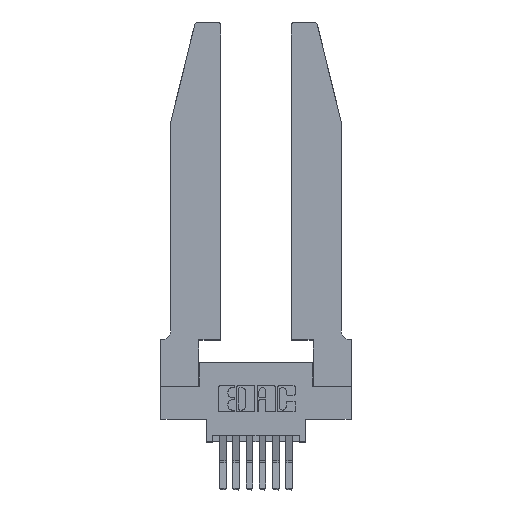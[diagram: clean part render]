
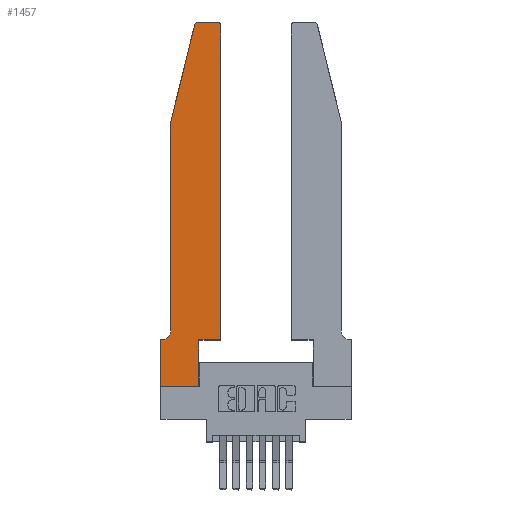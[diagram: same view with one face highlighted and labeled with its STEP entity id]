
A CAD part, top view. The second image highlights one B-rep face of the part: STEP entity #1457.
In plain terms, the highlighted planar face has unit normal (0, 0, 1).
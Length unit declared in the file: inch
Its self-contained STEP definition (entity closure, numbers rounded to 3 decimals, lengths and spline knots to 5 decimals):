
#40 = CARTESIAN_POINT ( 'NONE',  ( 0.2865, 0.35, 0.37 ) ) ;
#270 = VECTOR ( 'NONE', #13440, 39.37008 ) ;
#539 = EDGE_CURVE ( 'NONE', #5631, #12162, #7547, .T. ) ;
#817 = EDGE_CURVE ( 'NONE', #2137, #12603, #7372, .T. ) ;
#1002 = EDGE_CURVE ( 'NONE', #5883, #2137, #11207, .T. ) ;
#1016 = FACE_OUTER_BOUND ( 'NONE', #14484, .T. ) ;
#1052 = AXIS2_PLACEMENT_3D ( 'NONE', #11896, #5185, #13022 ) ;
#1059 = ORIENTED_EDGE ( 'NONE', *, *, #13550, .T. ) ;
#1457 = ADVANCED_FACE ( 'NONE', ( #1016 ), #13391, .T. ) ;
#1832 = CARTESIAN_POINT ( 'NONE',  ( 0., 0., 0.37 ) ) ;
#2078 = CIRCLE ( 'NONE', #1052, 0.03 ) ;
#2098 = DIRECTION ( 'NONE',  ( 0., 0., 1. ) ) ;
#2137 = VERTEX_POINT ( 'NONE', #9943 ) ;
#2771 = EDGE_CURVE ( 'NONE', #5979, #12823, #2805, .T. ) ;
#2805 = LINE ( 'NONE', #4105, #14296 ) ;
#3037 = VECTOR ( 'NONE', #4984, 39.37008 ) ;
#3042 = ORIENTED_EDGE ( 'NONE', *, *, #12965, .T. ) ;
#3043 = LINE ( 'NONE', #6247, #8605 ) ;
#3087 = ORIENTED_EDGE ( 'NONE', *, *, #8734, .T. ) ;
#3694 = CARTESIAN_POINT ( 'NONE',  ( 0.0755, 2., 0.37 ) ) ;
#3719 = DIRECTION ( 'NONE',  ( 0., 0., -1. ) ) ;
#3932 = VERTEX_POINT ( 'NONE', #12540 ) ;
#4089 = ORIENTED_EDGE ( 'NONE', *, *, #817, .T. ) ;
#4105 = CARTESIAN_POINT ( 'NONE',  ( 0.2605, 2.75, 0.37 ) ) ;
#4128 = ORIENTED_EDGE ( 'NONE', *, *, #5196, .T. ) ;
#4588 = DIRECTION ( 'NONE',  ( 0., 1., 0. ) ) ;
#4806 = VECTOR ( 'NONE', #6702, 39.37008 ) ;
#4925 = VECTOR ( 'NONE', #13739, 39.37008 ) ;
#4984 = DIRECTION ( 'NONE',  ( 1., 0., 0. ) ) ;
#5185 = DIRECTION ( 'NONE',  ( 0., 0., 1. ) ) ;
#5196 = EDGE_CURVE ( 'NONE', #12603, #14358, #13376, .T. ) ;
#5397 = LINE ( 'NONE', #13038, #11345 ) ;
#5611 = CARTESIAN_POINT ( 'NONE',  ( 0.0755, 0.35, 0.37 ) ) ;
#5631 = VERTEX_POINT ( 'NONE', #12059 ) ;
#5692 = CARTESIAN_POINT ( 'NONE',  ( 0.4505, 0.35, 0.37 ) ) ;
#5760 = ORIENTED_EDGE ( 'NONE', *, *, #7942, .T. ) ;
#5883 = VERTEX_POINT ( 'NONE', #6882 ) ;
#5979 = VERTEX_POINT ( 'NONE', #12626 ) ;
#6247 = CARTESIAN_POINT ( 'NONE',  ( 0.0755, 2., 0.37 ) ) ;
#6317 = DIRECTION ( 'NONE',  ( 0., -1., 0. ) ) ;
#6677 = VECTOR ( 'NONE', #7545, 39.37008 ) ;
#6678 = ORIENTED_EDGE ( 'NONE', *, *, #11827, .T. ) ;
#6702 = DIRECTION ( 'NONE',  ( 1., 0., 0. ) ) ;
#6876 = DIRECTION ( 'NONE',  ( -1., 0., 0. ) ) ;
#6882 = CARTESIAN_POINT ( 'NONE',  ( 0., 0., 0.37 ) ) ;
#6892 = EDGE_CURVE ( 'NONE', #14358, #3932, #7042, .T. ) ;
#7042 = LINE ( 'NONE', #9741, #6677 ) ;
#7162 = CIRCLE ( 'NONE', #13261, 0.07 ) ;
#7372 = LINE ( 'NONE', #9482, #13647 ) ;
#7545 = DIRECTION ( 'NONE',  ( 0., 1., 0. ) ) ;
#7547 = LINE ( 'NONE', #14328, #4925 ) ;
#7942 = EDGE_CURVE ( 'NONE', #12162, #8428, #3043, .T. ) ;
#8428 = VERTEX_POINT ( 'NONE', #12704 ) ;
#8605 = VECTOR ( 'NONE', #11840, 39.37008 ) ;
#8734 = EDGE_CURVE ( 'NONE', #3932, #5979, #13299, .T. ) ;
#8772 = CARTESIAN_POINT ( 'NONE',  ( 0.4205, 2.72, 0.37 ) ) ;
#8900 = LINE ( 'NONE', #5611, #270 ) ;
#9217 = VERTEX_POINT ( 'NONE', #13025 ) ;
#9385 = EDGE_CURVE ( 'NONE', #14176, #9217, #8900, .T. ) ;
#9410 = ORIENTED_EDGE ( 'NONE', *, *, #539, .T. ) ;
#9482 = CARTESIAN_POINT ( 'NONE',  ( 0.2865, 0.35, 0.37 ) ) ;
#9741 = CARTESIAN_POINT ( 'NONE',  ( 0.4505, 0.35, 0.37 ) ) ;
#9898 = DIRECTION ( 'NONE',  ( 1., 0., 0. ) ) ;
#9943 = CARTESIAN_POINT ( 'NONE',  ( 0.2865, 0., 0.37 ) ) ;
#10378 = CARTESIAN_POINT ( 'NONE',  ( 0.0055, 0.42, 0.37 ) ) ;
#11017 = ORIENTED_EDGE ( 'NONE', *, *, #9385, .T. ) ;
#11207 = LINE ( 'NONE', #1832, #3037 ) ;
#11345 = VECTOR ( 'NONE', #6317, 39.37008 ) ;
#11359 = DIRECTION ( 'NONE',  ( 0., 0., 1. ) ) ;
#11527 = DIRECTION ( 'NONE',  ( -1., 0., 0. ) ) ;
#11554 = AXIS2_PLACEMENT_3D ( 'NONE', #8772, #2098, #9898 ) ;
#11657 = DIRECTION ( 'NONE',  ( 1., 0., 0. ) ) ;
#11827 = EDGE_CURVE ( 'NONE', #8428, #14176, #7162, .T. ) ;
#11840 = DIRECTION ( 'NONE',  ( 0., -1., 0. ) ) ;
#11896 = CARTESIAN_POINT ( 'NONE',  ( 0.284, 2.72, 0.37 ) ) ;
#12059 = CARTESIAN_POINT ( 'NONE',  ( 0.25487, 2.72718, 0.37 ) ) ;
#12162 = VERTEX_POINT ( 'NONE', #3694 ) ;
#12503 = CARTESIAN_POINT ( 'NONE',  ( 0.4505, 0.35, 0.37 ) ) ;
#12540 = CARTESIAN_POINT ( 'NONE',  ( 0.4505, 2.72, 0.37 ) ) ;
#12562 = ORIENTED_EDGE ( 'NONE', *, *, #2771, .T. ) ;
#12603 = VERTEX_POINT ( 'NONE', #40 ) ;
#12626 = CARTESIAN_POINT ( 'NONE',  ( 0.4205, 2.75, 0.37 ) ) ;
#12663 = ORIENTED_EDGE ( 'NONE', *, *, #1002, .T. ) ;
#12704 = CARTESIAN_POINT ( 'NONE',  ( 0.0755, 0.42, 0.37 ) ) ;
#12800 = CARTESIAN_POINT ( 'NONE',  ( 0.284, 2.75, 0.37 ) ) ;
#12823 = VERTEX_POINT ( 'NONE', #12800 ) ;
#12965 = EDGE_CURVE ( 'NONE', #9217, #5883, #5397, .T. ) ;
#13022 = DIRECTION ( 'NONE',  ( 1., 0., 0. ) ) ;
#13025 = CARTESIAN_POINT ( 'NONE',  ( 0., 0.35, 0.37 ) ) ;
#13038 = CARTESIAN_POINT ( 'NONE',  ( 0., 0., 0.37 ) ) ;
#13241 = ORIENTED_EDGE ( 'NONE', *, *, #6892, .T. ) ;
#13261 = AXIS2_PLACEMENT_3D ( 'NONE', #10378, #3719, #11527 ) ;
#13299 = CIRCLE ( 'NONE', #11554, 0.03 ) ;
#13376 = LINE ( 'NONE', #12503, #4806 ) ;
#13391 = PLANE ( 'NONE',  #13435 ) ;
#13435 = AXIS2_PLACEMENT_3D ( 'NONE', #13439, #11359, #11657 ) ;
#13439 = CARTESIAN_POINT ( 'NONE',  ( 0., 0.35, 0.37 ) ) ;
#13440 = DIRECTION ( 'NONE',  ( -1., 0., 0. ) ) ;
#13550 = EDGE_CURVE ( 'NONE', #12823, #5631, #2078, .T. ) ;
#13647 = VECTOR ( 'NONE', #4588, 39.37008 ) ;
#13739 = DIRECTION ( 'NONE',  ( -0.239, -0.971, 0. ) ) ;
#14107 = CARTESIAN_POINT ( 'NONE',  ( 0.0055, 0.35, 0.37 ) ) ;
#14176 = VERTEX_POINT ( 'NONE', #14107 ) ;
#14296 = VECTOR ( 'NONE', #6876, 39.37008 ) ;
#14328 = CARTESIAN_POINT ( 'NONE',  ( 0.0755, 2., 0.37 ) ) ;
#14358 = VERTEX_POINT ( 'NONE', #5692 ) ;
#14484 = EDGE_LOOP ( 'NONE', ( #12562, #1059, #9410, #5760, #6678, #11017, #3042, #12663, #4089, #4128, #13241, #3087 ) ) ;
